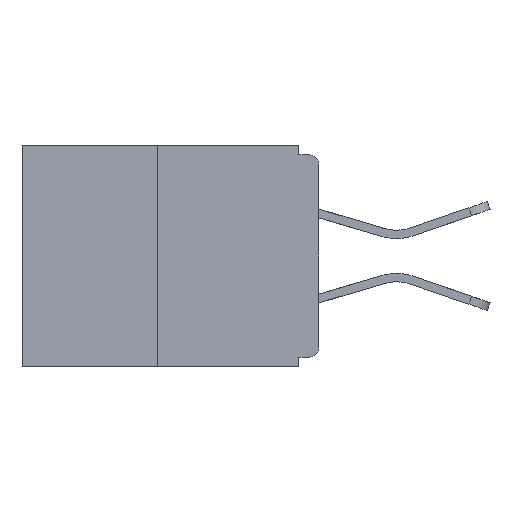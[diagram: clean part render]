
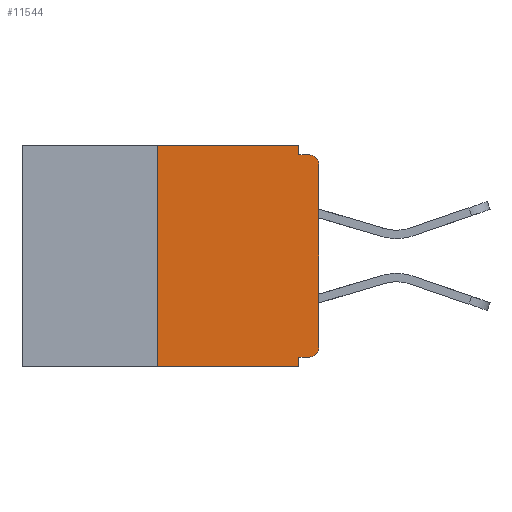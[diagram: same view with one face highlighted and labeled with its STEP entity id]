
A CAD part, left-side view. The second image highlights one B-rep face of the part: STEP entity #11544.
In plain terms, the highlighted planar face has unit normal (-1, 0, 0).
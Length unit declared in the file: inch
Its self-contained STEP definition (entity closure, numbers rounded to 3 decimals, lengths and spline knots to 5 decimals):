
#64 = CARTESIAN_POINT ( 'NONE',  ( 0., 0.015, -0.328 ) ) ;
#366 = ORIENTED_EDGE ( 'NONE', *, *, #11058, .T. ) ;
#658 = DIRECTION ( 'NONE',  ( 0., 0., -1. ) ) ;
#1059 = CARTESIAN_POINT ( 'NONE',  ( 0., 0.031, -0.328 ) ) ;
#1124 = AXIS2_PLACEMENT_3D ( 'NONE', #2071, #15157, #658 ) ;
#1163 = VERTEX_POINT ( 'NONE', #64 ) ;
#1267 = CARTESIAN_POINT ( 'NONE',  ( 0., 0.031, 0. ) ) ;
#1383 = EDGE_CURVE ( 'NONE', #5781, #17693, #9377, .T. ) ;
#1594 = AXIS2_PLACEMENT_3D ( 'NONE', #12101, #13586, #13400 ) ;
#1796 = DIRECTION ( 'NONE',  ( 0., 0., 1. ) ) ;
#1959 = ORIENTED_EDGE ( 'NONE', *, *, #14338, .T. ) ;
#2071 = CARTESIAN_POINT ( 'NONE',  ( 0., 0.015, -0.313 ) ) ;
#2650 = CARTESIAN_POINT ( 'NONE',  ( 0., 0.46, 0. ) ) ;
#2704 = VECTOR ( 'NONE', #15275, 39.37008 ) ;
#2903 = DIRECTION ( 'NONE',  ( 0., 0., 1. ) ) ;
#2922 = CARTESIAN_POINT ( 'NONE',  ( 0., 0., 0. ) ) ;
#3416 = VERTEX_POINT ( 'NONE', #9380 ) ;
#3703 = PLANE ( 'NONE',  #12318 ) ;
#3990 = DIRECTION ( 'NONE',  ( 0., -1., 0. ) ) ;
#4578 = EDGE_LOOP ( 'NONE', ( #18442, #6565, #366, #18352, #13162, #9147, #1959, #10278, #8060, #6433 ) ) ;
#4671 = CARTESIAN_POINT ( 'NONE',  ( 0., 0.25, 0. ) ) ;
#4994 = LINE ( 'NONE', #13399, #5227 ) ;
#5030 = EDGE_CURVE ( 'NONE', #1163, #10434, #14794, .T. ) ;
#5172 = EDGE_CURVE ( 'NONE', #16239, #12512, #14119, .T. ) ;
#5227 = VECTOR ( 'NONE', #14857, 39.37008 ) ;
#5266 = LINE ( 'NONE', #6725, #18465 ) ;
#5775 = VECTOR ( 'NONE', #7864, 39.37008 ) ;
#5781 = VERTEX_POINT ( 'NONE', #15034 ) ;
#5863 = LINE ( 'NONE', #2650, #6769 ) ;
#6433 = ORIENTED_EDGE ( 'NONE', *, *, #1383, .F. ) ;
#6565 = ORIENTED_EDGE ( 'NONE', *, *, #12830, .F. ) ;
#6725 = CARTESIAN_POINT ( 'NONE',  ( 0., 0., -0.328 ) ) ;
#6726 = CARTESIAN_POINT ( 'NONE',  ( 0., 0.46, 0. ) ) ;
#6769 = VECTOR ( 'NONE', #3990, 39.37008 ) ;
#7062 = DIRECTION ( 'NONE',  ( 0., 0., -1. ) ) ;
#7225 = VECTOR ( 'NONE', #1796, 39.37008 ) ;
#7864 = DIRECTION ( 'NONE',  ( 0., -1., 0. ) ) ;
#7886 = EDGE_CURVE ( 'NONE', #1163, #16239, #5266, .T. ) ;
#7940 = VERTEX_POINT ( 'NONE', #15802 ) ;
#8060 = ORIENTED_EDGE ( 'NONE', *, *, #13947, .F. ) ;
#8163 = DIRECTION ( 'NONE',  ( 0., 1., 0. ) ) ;
#8200 = FACE_OUTER_BOUND ( 'NONE', #4578, .T. ) ;
#8349 = CIRCLE ( 'NONE', #1594, 0.015 ) ;
#8935 = VERTEX_POINT ( 'NONE', #14967 ) ;
#9147 = ORIENTED_EDGE ( 'NONE', *, *, #5030, .T. ) ;
#9377 = LINE ( 'NONE', #1267, #15665 ) ;
#9380 = CARTESIAN_POINT ( 'NONE',  ( 0., 0., -0.03 ) ) ;
#10069 = CARTESIAN_POINT ( 'NONE',  ( 0., 0.25, 0. ) ) ;
#10278 = ORIENTED_EDGE ( 'NONE', *, *, #13641, .T. ) ;
#10434 = VERTEX_POINT ( 'NONE', #12916 ) ;
#10778 = DIRECTION ( 'NONE',  ( 0., 0., -1. ) ) ;
#11058 = EDGE_CURVE ( 'NONE', #7940, #12512, #11822, .T. ) ;
#11544 = ADVANCED_FACE ( 'NONE', ( #8200 ), #3703, .F. ) ;
#11822 = LINE ( 'NONE', #17935, #5775 ) ;
#11957 = LINE ( 'NONE', #2922, #7225 ) ;
#12101 = CARTESIAN_POINT ( 'NONE',  ( 0., 0.015, -0.03 ) ) ;
#12209 = VECTOR ( 'NONE', #2903, 39.37008 ) ;
#12318 = AXIS2_PLACEMENT_3D ( 'NONE', #6726, #13804, #10778 ) ;
#12512 = VERTEX_POINT ( 'NONE', #13735 ) ;
#12830 = EDGE_CURVE ( 'NONE', #7940, #18252, #15337, .T. ) ;
#12916 = CARTESIAN_POINT ( 'NONE',  ( 0., 0., -0.313 ) ) ;
#13162 = ORIENTED_EDGE ( 'NONE', *, *, #7886, .F. ) ;
#13399 = CARTESIAN_POINT ( 'NONE',  ( 0., 0., -0.015 ) ) ;
#13400 = DIRECTION ( 'NONE',  ( 0., 0., -1. ) ) ;
#13586 = DIRECTION ( 'NONE',  ( -1., 0., 0. ) ) ;
#13641 = EDGE_CURVE ( 'NONE', #3416, #8935, #8349, .T. ) ;
#13735 = CARTESIAN_POINT ( 'NONE',  ( 0., 0.031, -0.343 ) ) ;
#13804 = DIRECTION ( 'NONE',  ( 1., 0., 0. ) ) ;
#13947 = EDGE_CURVE ( 'NONE', #17693, #8935, #4994, .T. ) ;
#14119 = LINE ( 'NONE', #15214, #2704 ) ;
#14338 = EDGE_CURVE ( 'NONE', #10434, #3416, #11957, .T. ) ;
#14636 = EDGE_CURVE ( 'NONE', #18252, #5781, #5863, .T. ) ;
#14794 = CIRCLE ( 'NONE', #1124, 0.015 ) ;
#14857 = DIRECTION ( 'NONE',  ( 0., -1., 0. ) ) ;
#14967 = CARTESIAN_POINT ( 'NONE',  ( 0., 0.015, -0.015 ) ) ;
#15034 = CARTESIAN_POINT ( 'NONE',  ( 0., 0.031, 0. ) ) ;
#15157 = DIRECTION ( 'NONE',  ( -1., 0., 0. ) ) ;
#15214 = CARTESIAN_POINT ( 'NONE',  ( 0., 0.031, -0.343 ) ) ;
#15275 = DIRECTION ( 'NONE',  ( 0., 0., -1. ) ) ;
#15337 = LINE ( 'NONE', #10069, #12209 ) ;
#15665 = VECTOR ( 'NONE', #7062, 39.37008 ) ;
#15802 = CARTESIAN_POINT ( 'NONE',  ( 0., 0.25, -0.343 ) ) ;
#16239 = VERTEX_POINT ( 'NONE', #1059 ) ;
#16287 = CARTESIAN_POINT ( 'NONE',  ( 0., 0.031, -0.015 ) ) ;
#17693 = VERTEX_POINT ( 'NONE', #16287 ) ;
#17935 = CARTESIAN_POINT ( 'NONE',  ( 0., 0.46, -0.343 ) ) ;
#18252 = VERTEX_POINT ( 'NONE', #4671 ) ;
#18352 = ORIENTED_EDGE ( 'NONE', *, *, #5172, .F. ) ;
#18442 = ORIENTED_EDGE ( 'NONE', *, *, #14636, .F. ) ;
#18465 = VECTOR ( 'NONE', #8163, 39.37008 ) ;
